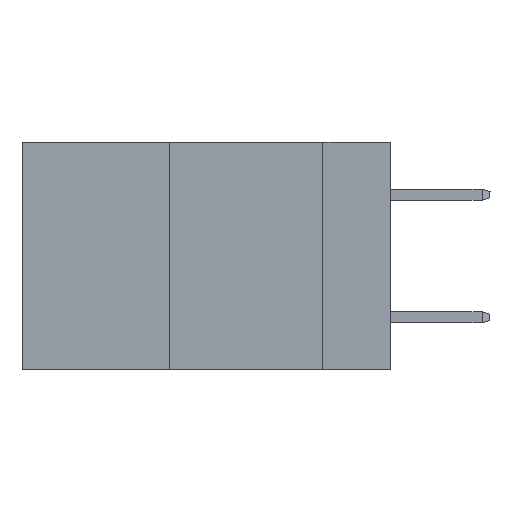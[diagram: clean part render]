
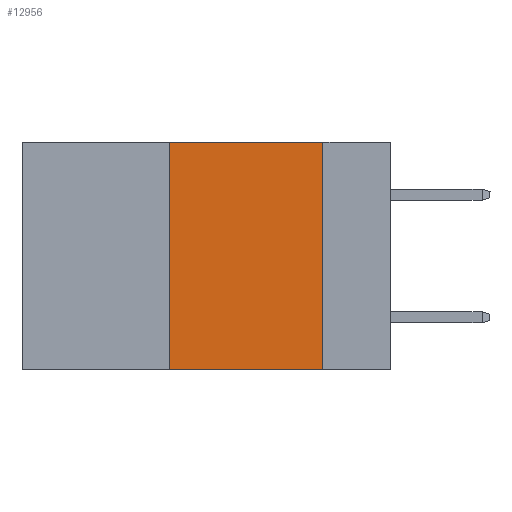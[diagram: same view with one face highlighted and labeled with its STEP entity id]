
A CAD part, left-side view. The second image highlights one B-rep face of the part: STEP entity #12956.
In plain terms, the highlighted planar face has unit normal (-1, 0, 0).
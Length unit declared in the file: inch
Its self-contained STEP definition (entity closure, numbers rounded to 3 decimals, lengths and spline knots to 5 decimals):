
#695 = FACE_OUTER_BOUND ( 'NONE', #10312, .T. ) ;
#1053 = CARTESIAN_POINT ( 'NONE',  ( 0., 0.11, -0.37 ) ) ;
#2220 = CARTESIAN_POINT ( 'NONE',  ( 0., 0.11, 0. ) ) ;
#2245 = VECTOR ( 'NONE', #5998, 39.37008 ) ;
#2529 = CARTESIAN_POINT ( 'NONE',  ( 0., 0.36, -0.37 ) ) ;
#2813 = VECTOR ( 'NONE', #4899, 39.37008 ) ;
#3401 = DIRECTION ( 'NONE',  ( 0., 0., -1. ) ) ;
#4899 = DIRECTION ( 'NONE',  ( 0., 0., -1. ) ) ;
#5036 = AXIS2_PLACEMENT_3D ( 'NONE', #12792, #10256, #3401 ) ;
#5998 = DIRECTION ( 'NONE',  ( 0., -1., 0. ) ) ;
#6046 = CARTESIAN_POINT ( 'NONE',  ( 0., 0.11, 0. ) ) ;
#6211 = LINE ( 'NONE', #6046, #2813 ) ;
#6265 = VERTEX_POINT ( 'NONE', #2529 ) ;
#7623 = LINE ( 'NONE', #15516, #16667 ) ;
#7966 = EDGE_CURVE ( 'NONE', #6265, #9495, #7623, .T. ) ;
#8901 = LINE ( 'NONE', #14260, #2245 ) ;
#9105 = CARTESIAN_POINT ( 'NONE',  ( 0., 0.6, -0.37 ) ) ;
#9495 = VERTEX_POINT ( 'NONE', #9496 ) ;
#9496 = CARTESIAN_POINT ( 'NONE',  ( 0., 0.36, 0. ) ) ;
#10137 = ORIENTED_EDGE ( 'NONE', *, *, #11871, .T. ) ;
#10256 = DIRECTION ( 'NONE',  ( 1., 0., 0. ) ) ;
#10312 = EDGE_LOOP ( 'NONE', ( #12404, #13410, #10347, #10137 ) ) ;
#10347 = ORIENTED_EDGE ( 'NONE', *, *, #7966, .F. ) ;
#10597 = LINE ( 'NONE', #9105, #12348 ) ;
#11339 = VERTEX_POINT ( 'NONE', #1053 ) ;
#11491 = DIRECTION ( 'NONE',  ( 0., 0., 1. ) ) ;
#11563 = PLANE ( 'NONE',  #5036 ) ;
#11871 = EDGE_CURVE ( 'NONE', #6265, #11339, #10597, .T. ) ;
#12348 = VECTOR ( 'NONE', #14527, 39.37008 ) ;
#12404 = ORIENTED_EDGE ( 'NONE', *, *, #13640, .F. ) ;
#12792 = CARTESIAN_POINT ( 'NONE',  ( 0., 0.6, 0. ) ) ;
#12956 = ADVANCED_FACE ( 'NONE', ( #695 ), #11563, .F. ) ;
#13410 = ORIENTED_EDGE ( 'NONE', *, *, #13473, .F. ) ;
#13473 = EDGE_CURVE ( 'NONE', #9495, #14682, #8901, .T. ) ;
#13640 = EDGE_CURVE ( 'NONE', #14682, #11339, #6211, .T. ) ;
#14260 = CARTESIAN_POINT ( 'NONE',  ( 0., 0.6, 0. ) ) ;
#14527 = DIRECTION ( 'NONE',  ( 0., -1., 0. ) ) ;
#14682 = VERTEX_POINT ( 'NONE', #2220 ) ;
#15516 = CARTESIAN_POINT ( 'NONE',  ( 0., 0.36, 0. ) ) ;
#16667 = VECTOR ( 'NONE', #11491, 39.37008 ) ;
